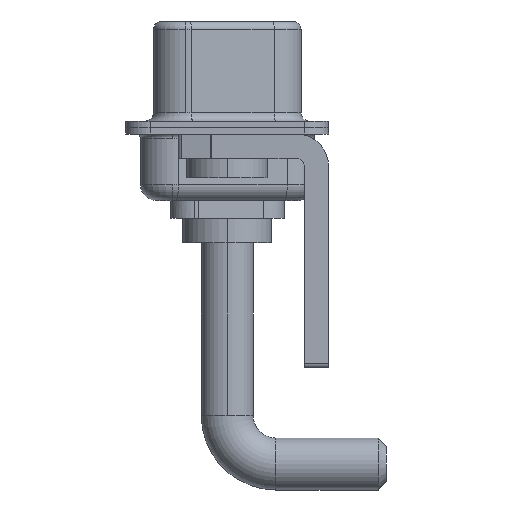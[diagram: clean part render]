
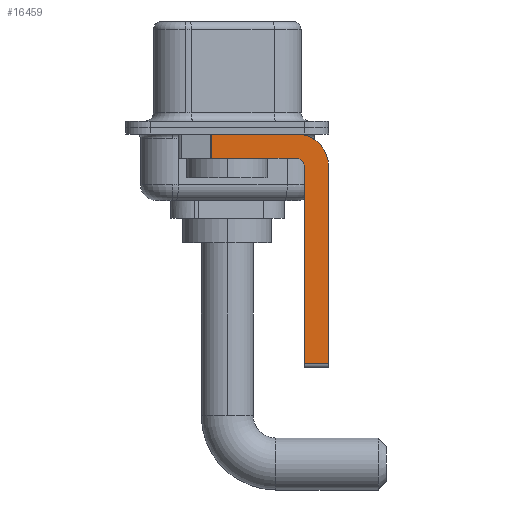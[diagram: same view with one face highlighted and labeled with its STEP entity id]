
A CAD part, left-side view. The second image highlights one B-rep face of the part: STEP entity #16459.
In plain terms, the highlighted planar face has unit normal (-1, 0, 0).
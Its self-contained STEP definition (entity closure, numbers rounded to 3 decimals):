
#128 = CARTESIAN_POINT ( 'NONE',  ( -2.9, 0.978, -0.4 ) ) ;
#602 = VERTEX_POINT ( 'NONE', #8411 ) ;
#618 = VERTEX_POINT ( 'NONE', #12471 ) ;
#1255 = EDGE_CURVE ( 'NONE', #10399, #602, #14155, .T. ) ;
#1362 = DIRECTION ( 'NONE',  ( 0., 0., -1. ) ) ;
#2180 = VECTOR ( 'NONE', #12477, 1000. ) ;
#2768 = CARTESIAN_POINT ( 'NONE',  ( -2.9, -4.25, -2.4 ) ) ;
#2810 = LINE ( 'NONE', #4107, #7242 ) ;
#2862 = CIRCLE ( 'NONE', #14435, 0.5 ) ;
#2918 = CARTESIAN_POINT ( 'NONE',  ( -2.9, -4.25, -1.9 ) ) ;
#2971 = EDGE_CURVE ( 'NONE', #15539, #618, #13516, .T. ) ;
#3428 = ORIENTED_EDGE ( 'NONE', *, *, #6012, .T. ) ;
#3533 = VECTOR ( 'NONE', #16751, 1000. ) ;
#3628 = CARTESIAN_POINT ( 'NONE',  ( -2.9, 3., -0.4 ) ) ;
#4107 = CARTESIAN_POINT ( 'NONE',  ( -2.9, 0.978, -1.9 ) ) ;
#4218 = CARTESIAN_POINT ( 'NONE',  ( -2.9, -4.25, -1.9 ) ) ;
#4379 = LINE ( 'NONE', #13930, #2180 ) ;
#5139 = ORIENTED_EDGE ( 'NONE', *, *, #15682, .F. ) ;
#5143 = DIRECTION ( 'NONE',  ( -1., 0., 0. ) ) ;
#5233 = ORIENTED_EDGE ( 'NONE', *, *, #12200, .T. ) ;
#5244 = DIRECTION ( 'NONE',  ( 0., -1., 0. ) ) ;
#5273 = FACE_OUTER_BOUND ( 'NONE', #10211, .T. ) ;
#5324 = CARTESIAN_POINT ( 'NONE',  ( -2.9, -6.25, -2.4 ) ) ;
#5915 = EDGE_CURVE ( 'NONE', #602, #15539, #6934, .T. ) ;
#5933 = ORIENTED_EDGE ( 'NONE', *, *, #5915, .F. ) ;
#6012 = EDGE_CURVE ( 'NONE', #15929, #618, #12997, .T. ) ;
#6113 = AXIS2_PLACEMENT_3D ( 'NONE', #8007, #12061, #1362 ) ;
#6536 = CARTESIAN_POINT ( 'NONE',  ( -2.9, -4.25, -14.55 ) ) ;
#6611 = DIRECTION ( 'NONE',  ( 0., 0., -1. ) ) ;
#6741 = DIRECTION ( 'NONE',  ( 0., 0., -1. ) ) ;
#6896 = ORIENTED_EDGE ( 'NONE', *, *, #10056, .F. ) ;
#6934 = CIRCLE ( 'NONE', #6113, 2. ) ;
#7242 = VECTOR ( 'NONE', #9380, 1000. ) ;
#7907 = CARTESIAN_POINT ( 'NONE',  ( -2.9, -4.75, -14.55 ) ) ;
#7989 = VECTOR ( 'NONE', #6611, 1000. ) ;
#8007 = CARTESIAN_POINT ( 'NONE',  ( -2.9, -4.25, -2.4 ) ) ;
#8122 = VERTEX_POINT ( 'NONE', #11619 ) ;
#8165 = ORIENTED_EDGE ( 'NONE', *, *, #13936, .F. ) ;
#8411 = CARTESIAN_POINT ( 'NONE',  ( -2.9, -4.25, -0.4 ) ) ;
#8891 = CARTESIAN_POINT ( 'NONE',  ( -2.9, -4.75, -2.4 ) ) ;
#9380 = DIRECTION ( 'NONE',  ( 0., 0., -1. ) ) ;
#10056 = EDGE_CURVE ( 'NONE', #15929, #15353, #4379, .T. ) ;
#10211 = EDGE_LOOP ( 'NONE', ( #15729, #5233, #5139, #8165, #6896, #3428, #12192, #5933 ) ) ;
#10399 = VERTEX_POINT ( 'NONE', #128 ) ;
#11221 = CARTESIAN_POINT ( 'NONE',  ( -2.9, -4.25, -2.4 ) ) ;
#11619 = CARTESIAN_POINT ( 'NONE',  ( -2.9, 0.978, -1.9 ) ) ;
#11717 = CARTESIAN_POINT ( 'NONE',  ( -2.9, -6.25, -2.4 ) ) ;
#11997 = DIRECTION ( 'NONE',  ( 1., 0., 0. ) ) ;
#12061 = DIRECTION ( 'NONE',  ( 1., 0., 0. ) ) ;
#12192 = ORIENTED_EDGE ( 'NONE', *, *, #2971, .F. ) ;
#12200 = EDGE_CURVE ( 'NONE', #10399, #8122, #2810, .T. ) ;
#12471 = CARTESIAN_POINT ( 'NONE',  ( -2.9, -6.25, -14.55 ) ) ;
#12477 = DIRECTION ( 'NONE',  ( 0., 0., 1. ) ) ;
#12575 = VECTOR ( 'NONE', #13442, 1000. ) ;
#12997 = LINE ( 'NONE', #6536, #13578 ) ;
#13442 = DIRECTION ( 'NONE',  ( 0., 1., 0. ) ) ;
#13516 = LINE ( 'NONE', #5324, #7989 ) ;
#13578 = VECTOR ( 'NONE', #5244, 1000. ) ;
#13682 = AXIS2_PLACEMENT_3D ( 'NONE', #2768, #11997, #6741 ) ;
#13803 = DIRECTION ( 'NONE',  ( 0., 0., 1. ) ) ;
#13930 = CARTESIAN_POINT ( 'NONE',  ( -2.9, -4.75, -14.8 ) ) ;
#13936 = EDGE_CURVE ( 'NONE', #15353, #15678, #2862, .T. ) ;
#14155 = LINE ( 'NONE', #3628, #3533 ) ;
#14435 = AXIS2_PLACEMENT_3D ( 'NONE', #11221, #5143, #13803 ) ;
#14592 = PLANE ( 'NONE',  #13682 ) ;
#14739 = LINE ( 'NONE', #2918, #12575 ) ;
#15353 = VERTEX_POINT ( 'NONE', #8891 ) ;
#15539 = VERTEX_POINT ( 'NONE', #11717 ) ;
#15678 = VERTEX_POINT ( 'NONE', #4218 ) ;
#15682 = EDGE_CURVE ( 'NONE', #15678, #8122, #14739, .T. ) ;
#15729 = ORIENTED_EDGE ( 'NONE', *, *, #1255, .F. ) ;
#15929 = VERTEX_POINT ( 'NONE', #7907 ) ;
#16459 = ADVANCED_FACE ( 'NONE', ( #5273 ), #14592, .F. ) ;
#16751 = DIRECTION ( 'NONE',  ( 0., -1., 0. ) ) ;
